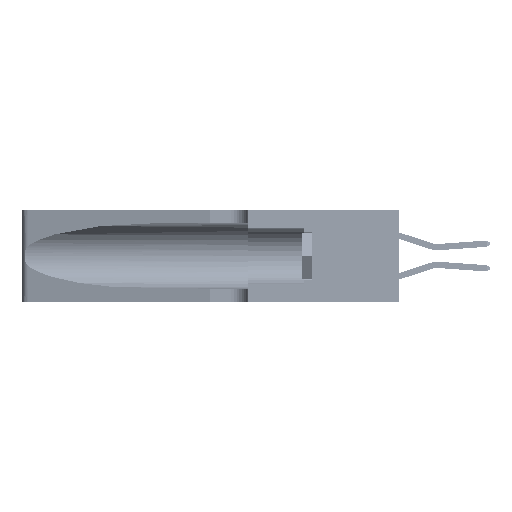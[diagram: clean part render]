
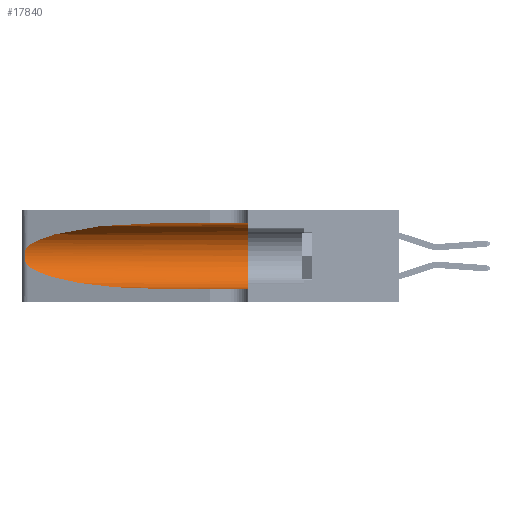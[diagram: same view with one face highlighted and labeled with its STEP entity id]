
A CAD part, left-side view. The second image highlights one B-rep face of the part: STEP entity #17840.
In plain terms, the highlighted cylindrical face has radius 3.308 mm (diameter 6.617 mm), a partial arc.
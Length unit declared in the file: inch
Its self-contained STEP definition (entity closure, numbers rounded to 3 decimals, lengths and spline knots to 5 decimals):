
#460 = FACE_OUTER_BOUND ( 'NONE', #36192, .T. ) ;
#1061 = CARTESIAN_POINT ( 'NONE',  ( 0.25487, 1.22718, 0.14631 ) ) ;
#2148 = ORIENTED_EDGE ( 'NONE', *, *, #45889, .T. ) ;
#2734 = CARTESIAN_POINT ( 'NONE',  ( 0.25856, 1.23593, 0.16098 ) ) ;
#3352 = EDGE_CURVE ( 'NONE', #33391, #40116, #4982, .T. ) ;
#3938 = CYLINDRICAL_SURFACE ( 'NONE', #22485, 0.13025 ) ;
#4982 = B_SPLINE_CURVE_WITH_KNOTS ( 'NONE', 3,
 ( #30107, #13390, #23996, #27807, #12755, #23839, #5511, #17221, #6311, #2734, #47034, #10136, #39324, #25073 ),
 .UNSPECIFIED., .F., .F.,
 ( 4, 2, 2, 2, 2, 2, 4 ),
 ( 0., 0.00027, 0.00053, 0.00107, 0.0016, 0.00187, 0.00214 ),
 .UNSPECIFIED. ) ;
#5511 = CARTESIAN_POINT ( 'NONE',  ( 0.26075, 1.23896, 0.19203 ) ) ;
#6311 = CARTESIAN_POINT ( 'NONE',  ( 0.26017, 1.23833, 0.17102 ) ) ;
#7243 = AXIS2_PLACEMENT_3D ( 'NONE', #21276, #35525, #43039 ) ;
#8540 =( BOUNDED_CURVE ( )  B_SPLINE_CURVE ( 3, ( #20093, #42177, #27614, #34511 ),
 .UNSPECIFIED., .F., .T. ) 
 B_SPLINE_CURVE_WITH_KNOTS ( ( 4, 4 ),
 ( 1.5708, 2.84003 ),
 .UNSPECIFIED. ) 
 CURVE ( )  GEOMETRIC_REPRESENTATION_ITEM ( )  RATIONAL_B_SPLINE_CURVE ( ( 1., 0.87, 0.87, 1. ) ) 
 REPRESENTATION_ITEM ( '' )  );
#10136 = CARTESIAN_POINT ( 'NONE',  ( 0.25639, 1.23186, 0.15144 ) ) ;
#10644 = CARTESIAN_POINT ( 'NONE',  ( 0.1305, 1.61858, 0.05475 ) ) ;
#10840 = VECTOR ( 'NONE', #47365, 39.37008 ) ;
#12755 = CARTESIAN_POINT ( 'NONE',  ( 0.25854, 1.2359, 0.20912 ) ) ;
#13029 = CARTESIAN_POINT ( 'NONE',  ( 0.25487, 1.22718, 0.14631 ) ) ;
#13390 = CARTESIAN_POINT ( 'NONE',  ( 0.25555, 1.22994, 0.2215 ) ) ;
#14151 =( BOUNDED_CURVE ( )  B_SPLINE_CURVE ( 3, ( #1061, #23731, #20008, #19861 ),
 .UNSPECIFIED., .F., .F. ) 
 B_SPLINE_CURVE_WITH_KNOTS ( ( 4, 4 ),
 ( 3.44316, 4.71239 ),
 .UNSPECIFIED. ) 
 CURVE ( )  GEOMETRIC_REPRESENTATION_ITEM ( )  RATIONAL_B_SPLINE_CURVE ( ( 1., 0.87, 0.87, 1. ) ) 
 REPRESENTATION_ITEM ( '' )  );
#14395 = EDGE_CURVE ( 'NONE', #15867, #31567, #38149, .T. ) ;
#15841 = VECTOR ( 'NONE', #19546, 39.37008 ) ;
#15867 = VERTEX_POINT ( 'NONE', #20569 ) ;
#16839 = CIRCLE ( 'NONE', #7243, 0.13025 ) ;
#17221 = CARTESIAN_POINT ( 'NONE',  ( 0.26075, 1.23896, 0.178 ) ) ;
#17840 = ADVANCED_FACE ( 'NONE', ( #460 ), #3938, .F. ) ;
#18171 = EDGE_CURVE ( 'NONE', #24841, #44962, #46383, .T. ) ;
#19546 = DIRECTION ( 'NONE',  ( 0., -1., 0. ) ) ;
#19861 = CARTESIAN_POINT ( 'NONE',  ( 0.1305, 0.72297, 0.05475 ) ) ;
#20008 = CARTESIAN_POINT ( 'NONE',  ( 0.18966, 0.96281, 0.05475 ) ) ;
#20093 = CARTESIAN_POINT ( 'NONE',  ( 0.1305, 0.72297, 0.31525 ) ) ;
#20569 = CARTESIAN_POINT ( 'NONE',  ( 0.1305, 0.72297, 0.31525 ) ) ;
#21276 = CARTESIAN_POINT ( 'NONE',  ( 0.1305, 0.35, 0.185 ) ) ;
#21840 = ORIENTED_EDGE ( 'NONE', *, *, #14395, .F. ) ;
#22485 = AXIS2_PLACEMENT_3D ( 'NONE', #29720, #40910, #22669 ) ;
#22665 = CARTESIAN_POINT ( 'NONE',  ( 0.25487, 1.22718, 0.22369 ) ) ;
#22669 = DIRECTION ( 'NONE',  ( 0., 0., -1. ) ) ;
#22811 = EDGE_CURVE ( 'NONE', #31567, #44962, #16839, .T. ) ;
#22876 = ORIENTED_EDGE ( 'NONE', *, *, #22811, .F. ) ;
#23731 = CARTESIAN_POINT ( 'NONE',  ( 0.2373, 1.15595, 0.08982 ) ) ;
#23839 = CARTESIAN_POINT ( 'NONE',  ( 0.26018, 1.23835, 0.19895 ) ) ;
#23996 = CARTESIAN_POINT ( 'NONE',  ( 0.25639, 1.23184, 0.21858 ) ) ;
#24841 = VERTEX_POINT ( 'NONE', #32774 ) ;
#25073 = CARTESIAN_POINT ( 'NONE',  ( 0.25487, 1.22718, 0.14631 ) ) ;
#27614 = CARTESIAN_POINT ( 'NONE',  ( 0.2373, 1.15595, 0.28018 ) ) ;
#27619 = ORIENTED_EDGE ( 'NONE', *, *, #18171, .T. ) ;
#27807 = CARTESIAN_POINT ( 'NONE',  ( 0.25787, 1.23484, 0.2124 ) ) ;
#29720 = CARTESIAN_POINT ( 'NONE',  ( 0.1305, 1.61858, 0.185 ) ) ;
#30107 = CARTESIAN_POINT ( 'NONE',  ( 0.25487, 1.22718, 0.22369 ) ) ;
#31567 = VERTEX_POINT ( 'NONE', #42099 ) ;
#32145 = EDGE_CURVE ( 'NONE', #40116, #24841, #14151, .T. ) ;
#32774 = CARTESIAN_POINT ( 'NONE',  ( 0.1305, 0.72297, 0.05475 ) ) ;
#33391 = VERTEX_POINT ( 'NONE', #22665 ) ;
#33607 = CARTESIAN_POINT ( 'NONE',  ( 0.1305, 0.35, 0.05475 ) ) ;
#34511 = CARTESIAN_POINT ( 'NONE',  ( 0.25487, 1.22718, 0.22369 ) ) ;
#35525 = DIRECTION ( 'NONE',  ( 0., 1., 0. ) ) ;
#36192 = EDGE_LOOP ( 'NONE', ( #2148, #46082, #41818, #27619, #22876, #21840 ) ) ;
#37634 = CARTESIAN_POINT ( 'NONE',  ( 0.1305, 1.61858, 0.31525 ) ) ;
#38149 = LINE ( 'NONE', #37634, #15841 ) ;
#39324 = CARTESIAN_POINT ( 'NONE',  ( 0.25555, 1.22993, 0.14849 ) ) ;
#40116 = VERTEX_POINT ( 'NONE', #13029 ) ;
#40910 = DIRECTION ( 'NONE',  ( 0., -1., 0. ) ) ;
#41818 = ORIENTED_EDGE ( 'NONE', *, *, #32145, .T. ) ;
#42099 = CARTESIAN_POINT ( 'NONE',  ( 0.1305, 0.35, 0.31525 ) ) ;
#42177 = CARTESIAN_POINT ( 'NONE',  ( 0.18966, 0.96281, 0.31525 ) ) ;
#43039 = DIRECTION ( 'NONE',  ( 0., 0., 1. ) ) ;
#44962 = VERTEX_POINT ( 'NONE', #33607 ) ;
#45889 = EDGE_CURVE ( 'NONE', #15867, #33391, #8540, .T. ) ;
#46082 = ORIENTED_EDGE ( 'NONE', *, *, #3352, .T. ) ;
#46383 = LINE ( 'NONE', #10644, #10840 ) ;
#47034 = CARTESIAN_POINT ( 'NONE',  ( 0.25789, 1.23486, 0.15765 ) ) ;
#47365 = DIRECTION ( 'NONE',  ( 0., -1., 0. ) ) ;
